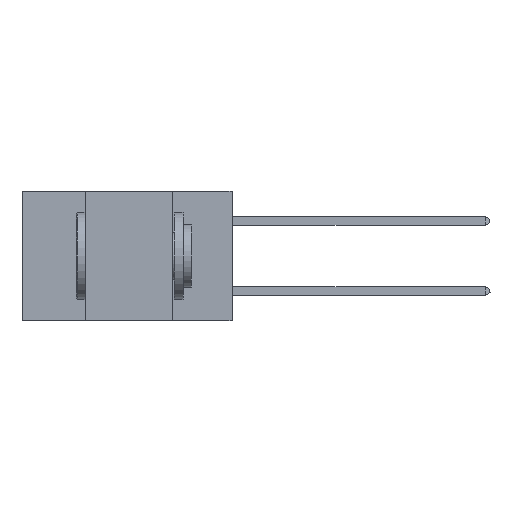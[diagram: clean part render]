
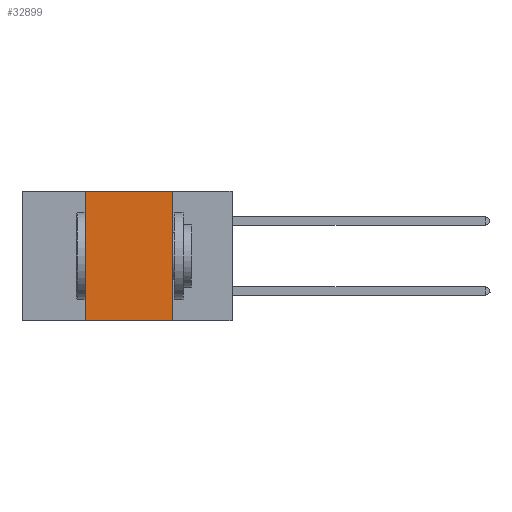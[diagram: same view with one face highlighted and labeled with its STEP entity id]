
A CAD part, left-side view. The second image highlights one B-rep face of the part: STEP entity #32899.
In plain terms, the highlighted planar face has unit normal (-1, 0, 0).
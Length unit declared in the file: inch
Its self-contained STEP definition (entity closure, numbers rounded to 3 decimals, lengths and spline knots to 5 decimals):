
#154 = CARTESIAN_POINT ( 'NONE',  ( 0., 0.42, 0. ) ) ;
#1594 = CARTESIAN_POINT ( 'NONE',  ( 0., 0.42, 0. ) ) ;
#2529 = VERTEX_POINT ( 'NONE', #17875 ) ;
#4737 = DIRECTION ( 'NONE',  ( 0., 0., -1. ) ) ;
#6123 = EDGE_CURVE ( 'NONE', #25490, #26005, #39190, .T. ) ;
#6201 = VECTOR ( 'NONE', #13700, 39.37008 ) ;
#6643 = VECTOR ( 'NONE', #21711, 39.37008 ) ;
#8672 = ORIENTED_EDGE ( 'NONE', *, *, #25079, .F. ) ;
#13562 = CARTESIAN_POINT ( 'NONE',  ( 0., 0.17, 0. ) ) ;
#13700 = DIRECTION ( 'NONE',  ( 0., 0., -1. ) ) ;
#14998 = VECTOR ( 'NONE', #37640, 39.37008 ) ;
#16973 = LINE ( 'NONE', #1594, #6643 ) ;
#17152 = CARTESIAN_POINT ( 'NONE',  ( 0., 0.17, 0. ) ) ;
#17376 = ORIENTED_EDGE ( 'NONE', *, *, #20692, .F. ) ;
#17875 = CARTESIAN_POINT ( 'NONE',  ( 0., 0.42, -0.37 ) ) ;
#18029 = VERTEX_POINT ( 'NONE', #154 ) ;
#20692 = EDGE_CURVE ( 'NONE', #2529, #18029, #16973, .T. ) ;
#21070 = FACE_OUTER_BOUND ( 'NONE', #26038, .T. ) ;
#21428 = DIRECTION ( 'NONE',  ( 0., -1., 0. ) ) ;
#21711 = DIRECTION ( 'NONE',  ( 0., 0., 1. ) ) ;
#22880 = CARTESIAN_POINT ( 'NONE',  ( 0., 0.17, -0.37 ) ) ;
#23099 = ORIENTED_EDGE ( 'NONE', *, *, #6123, .F. ) ;
#25079 = EDGE_CURVE ( 'NONE', #18029, #25490, #29892, .T. ) ;
#25490 = VERTEX_POINT ( 'NONE', #17152 ) ;
#26005 = VERTEX_POINT ( 'NONE', #22880 ) ;
#26038 = EDGE_LOOP ( 'NONE', ( #23099, #8672, #17376, #38887 ) ) ;
#27674 = CARTESIAN_POINT ( 'NONE',  ( 0., 0.6, 0. ) ) ;
#28045 = CARTESIAN_POINT ( 'NONE',  ( 0., 0.6, -0.37 ) ) ;
#28063 = EDGE_CURVE ( 'NONE', #2529, #26005, #39276, .T. ) ;
#29892 = LINE ( 'NONE', #27674, #14998 ) ;
#31161 = DIRECTION ( 'NONE',  ( 1., 0., 0. ) ) ;
#31483 = VECTOR ( 'NONE', #21428, 39.37008 ) ;
#32899 = ADVANCED_FACE ( 'NONE', ( #21070 ), #33885, .F. ) ;
#33885 = PLANE ( 'NONE',  #36822 ) ;
#36822 = AXIS2_PLACEMENT_3D ( 'NONE', #41167, #31161, #4737 ) ;
#37640 = DIRECTION ( 'NONE',  ( 0., -1., 0. ) ) ;
#38887 = ORIENTED_EDGE ( 'NONE', *, *, #28063, .T. ) ;
#39190 = LINE ( 'NONE', #13562, #6201 ) ;
#39276 = LINE ( 'NONE', #28045, #31483 ) ;
#41167 = CARTESIAN_POINT ( 'NONE',  ( 0., 0.6, 0. ) ) ;
